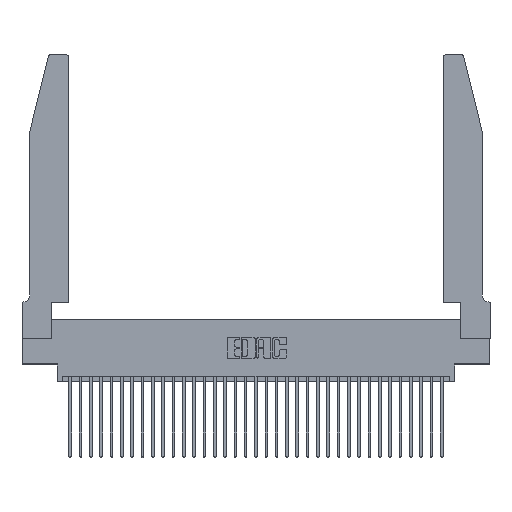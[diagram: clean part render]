
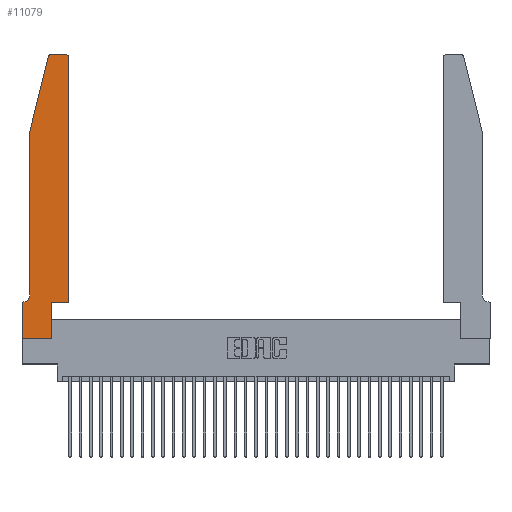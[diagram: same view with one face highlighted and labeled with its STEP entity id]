
A CAD part, top view. The second image highlights one B-rep face of the part: STEP entity #11079.
In plain terms, the highlighted planar face has unit normal (0, 0, 1).
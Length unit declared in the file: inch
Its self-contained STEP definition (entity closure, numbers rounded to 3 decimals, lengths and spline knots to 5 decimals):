
#140 = VERTEX_POINT ( 'NONE', #7237 ) ;
#615 = CARTESIAN_POINT ( 'NONE',  ( 0.4505, 0.35, 0.37 ) ) ;
#732 = ORIENTED_EDGE ( 'NONE', *, *, #25941, .T. ) ;
#976 = VERTEX_POINT ( 'NONE', #2581 ) ;
#1047 = DIRECTION ( 'NONE',  ( -1., 0., 0. ) ) ;
#1579 = VERTEX_POINT ( 'NONE', #26006 ) ;
#2256 = ORIENTED_EDGE ( 'NONE', *, *, #4668, .T. ) ;
#2538 = AXIS2_PLACEMENT_3D ( 'NONE', #11669, #22566, #1047 ) ;
#2581 = CARTESIAN_POINT ( 'NONE',  ( 0.4505, 0.35, 0.37 ) ) ;
#2669 = EDGE_CURVE ( 'NONE', #7444, #976, #15471, .T. ) ;
#3139 = LINE ( 'NONE', #8487, #22360 ) ;
#3160 = EDGE_CURVE ( 'NONE', #18397, #140, #6646, .T. ) ;
#3180 = DIRECTION ( 'NONE',  ( 0., 0., 1. ) ) ;
#3330 = LINE ( 'NONE', #18502, #30998 ) ;
#3658 = AXIS2_PLACEMENT_3D ( 'NONE', #19212, #3180, #8532 ) ;
#4045 = CARTESIAN_POINT ( 'NONE',  ( 0.25487, 2.72718, 0.37 ) ) ;
#4668 = EDGE_CURVE ( 'NONE', #7241, #7444, #14321, .T. ) ;
#4845 = CARTESIAN_POINT ( 'NONE',  ( 0.2865, 0.35, 0.37 ) ) ;
#4911 = CARTESIAN_POINT ( 'NONE',  ( 0., 0.35, 0.37 ) ) ;
#5155 = CARTESIAN_POINT ( 'NONE',  ( 0.0755, 0.35, 0.37 ) ) ;
#6117 = LINE ( 'NONE', #13305, #29607 ) ;
#6522 = CIRCLE ( 'NONE', #2538, 0.07 ) ;
#6540 = CARTESIAN_POINT ( 'NONE',  ( 0.0755, 2., 0.37 ) ) ;
#6548 = ORIENTED_EDGE ( 'NONE', *, *, #19511, .T. ) ;
#6603 = VECTOR ( 'NONE', #30447, 39.37008 ) ;
#6646 = CIRCLE ( 'NONE', #3658, 0.03 ) ;
#7056 = CIRCLE ( 'NONE', #13413, 0.03 ) ;
#7130 = EDGE_LOOP ( 'NONE', ( #732, #6548, #20880, #25820, #10874, #20739, #7925, #21695, #2256, #22289, #23346, #13632 ) ) ;
#7143 = VERTEX_POINT ( 'NONE', #4045 ) ;
#7237 = CARTESIAN_POINT ( 'NONE',  ( 0.4205, 2.75, 0.37 ) ) ;
#7241 = VERTEX_POINT ( 'NONE', #28393 ) ;
#7444 = VERTEX_POINT ( 'NONE', #4845 ) ;
#7874 = VECTOR ( 'NONE', #27851, 39.37008 ) ;
#7925 = ORIENTED_EDGE ( 'NONE', *, *, #21132, .T. ) ;
#8170 = DIRECTION ( 'NONE',  ( -1., 0., 0. ) ) ;
#8178 = DIRECTION ( 'NONE',  ( 0., -1., 0. ) ) ;
#8487 = CARTESIAN_POINT ( 'NONE',  ( 0., 0., 0.37 ) ) ;
#8532 = DIRECTION ( 'NONE',  ( 1., 0., 0. ) ) ;
#8751 = CARTESIAN_POINT ( 'NONE',  ( 0.2605, 2.75, 0.37 ) ) ;
#9916 = PLANE ( 'NONE',  #32535 ) ;
#9946 = LINE ( 'NONE', #8751, #7874 ) ;
#10332 = EDGE_CURVE ( 'NONE', #7143, #10459, #6117, .T. ) ;
#10435 = EDGE_CURVE ( 'NONE', #25903, #12847, #6522, .T. ) ;
#10459 = VERTEX_POINT ( 'NONE', #6540 ) ;
#10874 = ORIENTED_EDGE ( 'NONE', *, *, #10435, .T. ) ;
#11079 = ADVANCED_FACE ( 'NONE', ( #24485 ), #9916, .T. ) ;
#11336 = CARTESIAN_POINT ( 'NONE',  ( 0.0755, 0.42, 0.37 ) ) ;
#11669 = CARTESIAN_POINT ( 'NONE',  ( 0.0055, 0.42, 0.37 ) ) ;
#11708 = LINE ( 'NONE', #5155, #20121 ) ;
#12847 = VERTEX_POINT ( 'NONE', #19251 ) ;
#13305 = CARTESIAN_POINT ( 'NONE',  ( 0.0755, 2., 0.37 ) ) ;
#13413 = AXIS2_PLACEMENT_3D ( 'NONE', #20209, #25947, #28413 ) ;
#13612 = EDGE_CURVE ( 'NONE', #12847, #13777, #11708, .T. ) ;
#13632 = ORIENTED_EDGE ( 'NONE', *, *, #3160, .T. ) ;
#13777 = VERTEX_POINT ( 'NONE', #16876 ) ;
#14321 = LINE ( 'NONE', #20642, #20188 ) ;
#15471 = LINE ( 'NONE', #18650, #20041 ) ;
#15924 = DIRECTION ( 'NONE',  ( 0., -1., 0. ) ) ;
#16664 = CARTESIAN_POINT ( 'NONE',  ( 0., 0., 0.37 ) ) ;
#16829 = VECTOR ( 'NONE', #22385, 39.37008 ) ;
#16876 = CARTESIAN_POINT ( 'NONE',  ( 0., 0.35, 0.37 ) ) ;
#17151 = EDGE_CURVE ( 'NONE', #976, #18397, #31108, .T. ) ;
#18397 = VERTEX_POINT ( 'NONE', #28041 ) ;
#18502 = CARTESIAN_POINT ( 'NONE',  ( 0.0755, 2., 0.37 ) ) ;
#18650 = CARTESIAN_POINT ( 'NONE',  ( 0.4505, 0.35, 0.37 ) ) ;
#19212 = CARTESIAN_POINT ( 'NONE',  ( 0.4205, 2.72, 0.37 ) ) ;
#19251 = CARTESIAN_POINT ( 'NONE',  ( 0.0055, 0.35, 0.37 ) ) ;
#19511 = EDGE_CURVE ( 'NONE', #1579, #7143, #7056, .T. ) ;
#19869 = CARTESIAN_POINT ( 'NONE',  ( 0., 0., 0.37 ) ) ;
#20041 = VECTOR ( 'NONE', #27582, 39.37008 ) ;
#20121 = VECTOR ( 'NONE', #8170, 39.37008 ) ;
#20188 = VECTOR ( 'NONE', #26009, 39.37008 ) ;
#20209 = CARTESIAN_POINT ( 'NONE',  ( 0.284, 2.72, 0.37 ) ) ;
#20642 = CARTESIAN_POINT ( 'NONE',  ( 0.2865, 0.35, 0.37 ) ) ;
#20739 = ORIENTED_EDGE ( 'NONE', *, *, #13612, .T. ) ;
#20880 = ORIENTED_EDGE ( 'NONE', *, *, #10332, .T. ) ;
#21132 = EDGE_CURVE ( 'NONE', #13777, #28489, #3139, .T. ) ;
#21695 = ORIENTED_EDGE ( 'NONE', *, *, #33030, .T. ) ;
#22289 = ORIENTED_EDGE ( 'NONE', *, *, #2669, .T. ) ;
#22360 = VECTOR ( 'NONE', #8178, 39.37008 ) ;
#22385 = DIRECTION ( 'NONE',  ( 0., 1., 0. ) ) ;
#22566 = DIRECTION ( 'NONE',  ( 0., 0., -1. ) ) ;
#23346 = ORIENTED_EDGE ( 'NONE', *, *, #17151, .T. ) ;
#23849 = EDGE_CURVE ( 'NONE', #10459, #25903, #3330, .T. ) ;
#24485 = FACE_OUTER_BOUND ( 'NONE', #7130, .T. ) ;
#25820 = ORIENTED_EDGE ( 'NONE', *, *, #23849, .T. ) ;
#25903 = VERTEX_POINT ( 'NONE', #11336 ) ;
#25941 = EDGE_CURVE ( 'NONE', #140, #1579, #9946, .T. ) ;
#25947 = DIRECTION ( 'NONE',  ( 0., 0., 1. ) ) ;
#26006 = CARTESIAN_POINT ( 'NONE',  ( 0.284, 2.75, 0.37 ) ) ;
#26009 = DIRECTION ( 'NONE',  ( 0., 1., 0. ) ) ;
#26296 = DIRECTION ( 'NONE',  ( 0., 0., 1. ) ) ;
#27582 = DIRECTION ( 'NONE',  ( 1., 0., 0. ) ) ;
#27851 = DIRECTION ( 'NONE',  ( -1., 0., 0. ) ) ;
#28041 = CARTESIAN_POINT ( 'NONE',  ( 0.4505, 2.72, 0.37 ) ) ;
#28393 = CARTESIAN_POINT ( 'NONE',  ( 0.2865, 0., 0.37 ) ) ;
#28413 = DIRECTION ( 'NONE',  ( 1., 0., 0. ) ) ;
#28489 = VERTEX_POINT ( 'NONE', #19869 ) ;
#29220 = DIRECTION ( 'NONE',  ( -0.239, -0.971, 0. ) ) ;
#29607 = VECTOR ( 'NONE', #29220, 39.37008 ) ;
#30447 = DIRECTION ( 'NONE',  ( 1., 0., 0. ) ) ;
#30998 = VECTOR ( 'NONE', #15924, 39.37008 ) ;
#31108 = LINE ( 'NONE', #615, #16829 ) ;
#32535 = AXIS2_PLACEMENT_3D ( 'NONE', #4911, #26296, #34046 ) ;
#33030 = EDGE_CURVE ( 'NONE', #28489, #7241, #33883, .T. ) ;
#33883 = LINE ( 'NONE', #16664, #6603 ) ;
#34046 = DIRECTION ( 'NONE',  ( 1., 0., 0. ) ) ;
